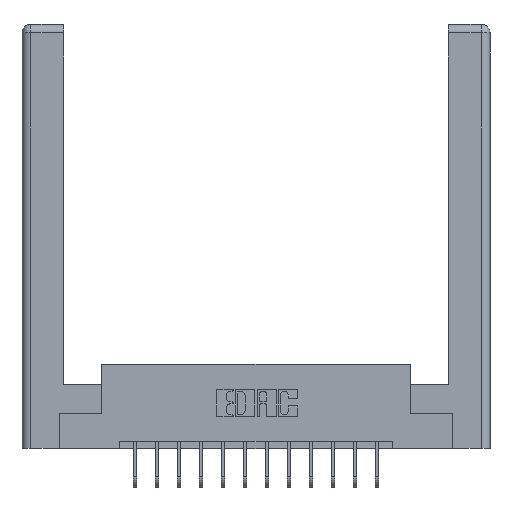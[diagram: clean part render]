
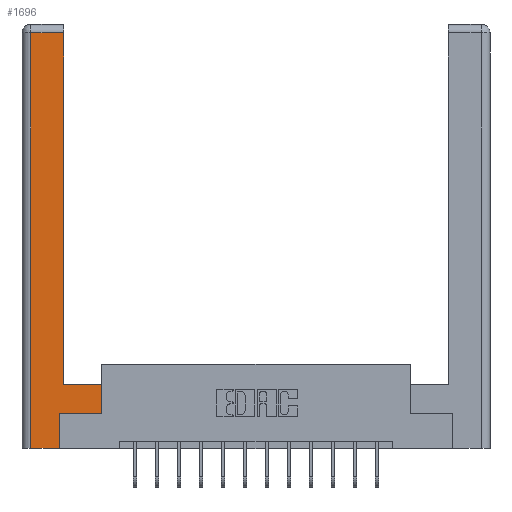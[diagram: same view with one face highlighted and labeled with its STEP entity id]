
A CAD part, top view. The second image highlights one B-rep face of the part: STEP entity #1696.
In plain terms, the highlighted planar face has unit normal (0, 0, 1).
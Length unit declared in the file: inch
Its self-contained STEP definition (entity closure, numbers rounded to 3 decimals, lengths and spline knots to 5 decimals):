
#43 = EDGE_CURVE ( 'NONE', #12733, #15066, #15484, .T. ) ;
#598 = ORIENTED_EDGE ( 'NONE', *, *, #5522, .T. ) ;
#671 = VERTEX_POINT ( 'NONE', #10974 ) ;
#1214 = CARTESIAN_POINT ( 'NONE',  ( 0.295, 3., 0. ) ) ;
#1295 = CARTESIAN_POINT ( 'NONE',  ( 0.265, 0.245, 0. ) ) ;
#1395 = CARTESIAN_POINT ( 'NONE',  ( 0.565, 0.245, 0. ) ) ;
#1529 = DIRECTION ( 'NONE',  ( -1., 0., 0. ) ) ;
#1592 = CARTESIAN_POINT ( 'NONE',  ( 0.265, 0., 0. ) ) ;
#1630 = DIRECTION ( 'NONE',  ( 0., 0., -1. ) ) ;
#1696 = ADVANCED_FACE ( 'NONE', ( #10935 ), #13413, .F. ) ;
#2286 = LINE ( 'NONE', #4304, #13510 ) ;
#2408 = DIRECTION ( 'NONE',  ( 0., 1., 0. ) ) ;
#2987 = CARTESIAN_POINT ( 'NONE',  ( 0.0615, 2.94, 0. ) ) ;
#3267 = EDGE_CURVE ( 'NONE', #15066, #6756, #14301, .T. ) ;
#3590 = LINE ( 'NONE', #1395, #14468 ) ;
#3869 = CARTESIAN_POINT ( 'NONE',  ( 0.0615, 0., 0. ) ) ;
#3871 = VECTOR ( 'NONE', #10791, 39.37008 ) ;
#3920 = ORIENTED_EDGE ( 'NONE', *, *, #14948, .T. ) ;
#4302 = ORIENTED_EDGE ( 'NONE', *, *, #10807, .T. ) ;
#4304 = CARTESIAN_POINT ( 'NONE',  ( 0.565, 0.45, 0. ) ) ;
#4787 = CARTESIAN_POINT ( 'NONE',  ( 0.295, 0.45, 0. ) ) ;
#5182 = VERTEX_POINT ( 'NONE', #10082 ) ;
#5405 = ORIENTED_EDGE ( 'NONE', *, *, #43, .T. ) ;
#5451 = VECTOR ( 'NONE', #5681, 39.37008 ) ;
#5469 = AXIS2_PLACEMENT_3D ( 'NONE', #14778, #1630, #1529 ) ;
#5522 = EDGE_CURVE ( 'NONE', #14602, #8843, #15540, .T. ) ;
#5681 = DIRECTION ( 'NONE',  ( 0., -1., 0. ) ) ;
#5824 = CARTESIAN_POINT ( 'NONE',  ( 0.0615, 0., 0. ) ) ;
#5948 = CARTESIAN_POINT ( 'NONE',  ( 0.265, 0., 0. ) ) ;
#6500 = DIRECTION ( 'NONE',  ( 1., 0., 0. ) ) ;
#6756 = VERTEX_POINT ( 'NONE', #14042 ) ;
#7287 = LINE ( 'NONE', #2987, #11794 ) ;
#7576 = DIRECTION ( 'NONE',  ( -1., 0., 0. ) ) ;
#7857 = CARTESIAN_POINT ( 'NONE',  ( 0.565, 0.45, 0. ) ) ;
#8268 = DIRECTION ( 'NONE',  ( 0., 1., 0. ) ) ;
#8390 = CARTESIAN_POINT ( 'NONE',  ( 0.265, 0.245, 0. ) ) ;
#8843 = VERTEX_POINT ( 'NONE', #1592 ) ;
#9987 = LINE ( 'NONE', #1295, #14315 ) ;
#10082 = CARTESIAN_POINT ( 'NONE',  ( 0.0615, 2.94, 0. ) ) ;
#10196 = ORIENTED_EDGE ( 'NONE', *, *, #11558, .T. ) ;
#10728 = VERTEX_POINT ( 'NONE', #8390 ) ;
#10791 = DIRECTION ( 'NONE',  ( -1., 0., 0. ) ) ;
#10807 = EDGE_CURVE ( 'NONE', #10728, #671, #3590, .T. ) ;
#10929 = CARTESIAN_POINT ( 'NONE',  ( 0.295, 0.45, 0. ) ) ;
#10935 = FACE_OUTER_BOUND ( 'NONE', #13074, .T. ) ;
#10974 = CARTESIAN_POINT ( 'NONE',  ( 0.565, 0.245, 0. ) ) ;
#11045 = EDGE_CURVE ( 'NONE', #671, #12733, #2286, .T. ) ;
#11202 = EDGE_CURVE ( 'NONE', #5182, #14602, #12945, .T. ) ;
#11558 = EDGE_CURVE ( 'NONE', #6756, #5182, #7287, .T. ) ;
#11794 = VECTOR ( 'NONE', #7576, 39.37008 ) ;
#12733 = VERTEX_POINT ( 'NONE', #7857 ) ;
#12803 = VECTOR ( 'NONE', #8268, 39.37008 ) ;
#12945 = LINE ( 'NONE', #5824, #5451 ) ;
#12956 = ORIENTED_EDGE ( 'NONE', *, *, #11202, .T. ) ;
#13074 = EDGE_LOOP ( 'NONE', ( #13820, #10196, #12956, #598, #3920, #4302, #14951, #5405 ) ) ;
#13413 = PLANE ( 'NONE',  #5469 ) ;
#13510 = VECTOR ( 'NONE', #13851, 39.37008 ) ;
#13820 = ORIENTED_EDGE ( 'NONE', *, *, #3267, .T. ) ;
#13851 = DIRECTION ( 'NONE',  ( 0., 1., 0. ) ) ;
#14042 = CARTESIAN_POINT ( 'NONE',  ( 0.295, 2.94, 0. ) ) ;
#14301 = LINE ( 'NONE', #1214, #12803 ) ;
#14315 = VECTOR ( 'NONE', #2408, 39.37008 ) ;
#14468 = VECTOR ( 'NONE', #6500, 39.37008 ) ;
#14602 = VERTEX_POINT ( 'NONE', #3869 ) ;
#14778 = CARTESIAN_POINT ( 'NONE',  ( 0., 0., 0. ) ) ;
#14804 = VECTOR ( 'NONE', #15095, 39.37008 ) ;
#14948 = EDGE_CURVE ( 'NONE', #8843, #10728, #9987, .T. ) ;
#14951 = ORIENTED_EDGE ( 'NONE', *, *, #11045, .T. ) ;
#15066 = VERTEX_POINT ( 'NONE', #10929 ) ;
#15095 = DIRECTION ( 'NONE',  ( 1., 0., 0. ) ) ;
#15484 = LINE ( 'NONE', #4787, #3871 ) ;
#15540 = LINE ( 'NONE', #5948, #14804 ) ;
